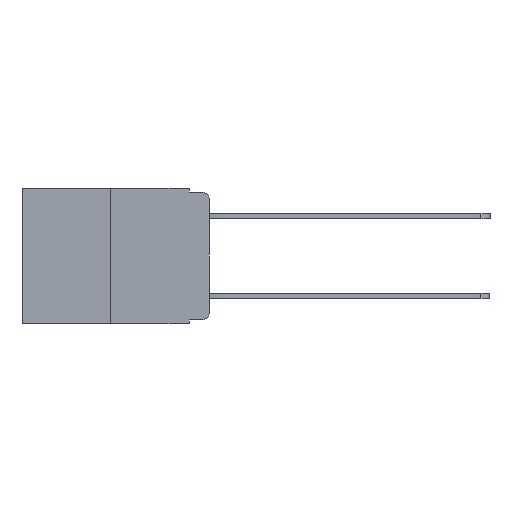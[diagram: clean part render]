
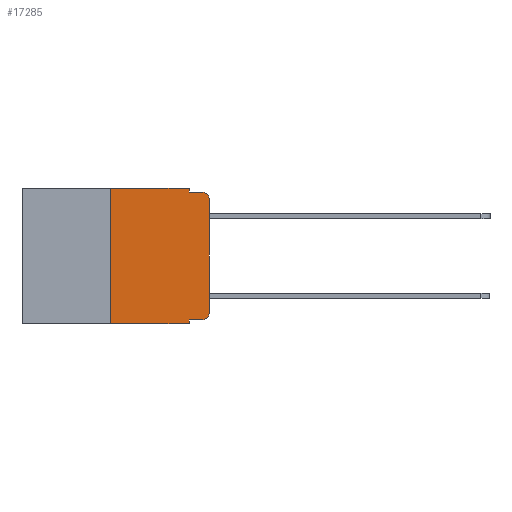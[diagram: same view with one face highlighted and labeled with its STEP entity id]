
A CAD part, left-side view. The second image highlights one B-rep face of the part: STEP entity #17285.
In plain terms, the highlighted planar face has unit normal (-1, 0, 0).
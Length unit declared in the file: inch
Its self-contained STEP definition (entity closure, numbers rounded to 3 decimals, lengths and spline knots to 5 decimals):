
#132 = DIRECTION ( 'NONE',  ( 0., -1., 0. ) ) ;
#447 = ORIENTED_EDGE ( 'NONE', *, *, #4931, .T. ) ;
#500 = VECTOR ( 'NONE', #19160, 39.37008 ) ;
#518 = CARTESIAN_POINT ( 'NONE',  ( 0., 0.02, -0.03 ) ) ;
#714 = ORIENTED_EDGE ( 'NONE', *, *, #6382, .F. ) ;
#965 = VERTEX_POINT ( 'NONE', #17814 ) ;
#993 = CARTESIAN_POINT ( 'NONE',  ( 0., 0.051, 0. ) ) ;
#1452 = VERTEX_POINT ( 'NONE', #8484 ) ;
#1464 = VECTOR ( 'NONE', #8050, 39.37008 ) ;
#2124 = ORIENTED_EDGE ( 'NONE', *, *, #16101, .T. ) ;
#2164 = DIRECTION ( 'NONE',  ( -1., 0., 0. ) ) ;
#2331 = DIRECTION ( 'NONE',  ( 0., 0., -1. ) ) ;
#3204 = EDGE_CURVE ( 'NONE', #4853, #1452, #14999, .T. ) ;
#3598 = LINE ( 'NONE', #10023, #22361 ) ;
#3828 = VERTEX_POINT ( 'NONE', #17256 ) ;
#4351 = ORIENTED_EDGE ( 'NONE', *, *, #3204, .F. ) ;
#4436 = CARTESIAN_POINT ( 'NONE',  ( 0., 0.051, 0. ) ) ;
#4838 = DIRECTION ( 'NONE',  ( 0., -1., 0. ) ) ;
#4853 = VERTEX_POINT ( 'NONE', #17505 ) ;
#4931 = EDGE_CURVE ( 'NONE', #15248, #3828, #8973, .T. ) ;
#4981 = CARTESIAN_POINT ( 'NONE',  ( 0., 0.473, 0. ) ) ;
#5122 = FACE_OUTER_BOUND ( 'NONE', #17758, .T. ) ;
#5472 = ORIENTED_EDGE ( 'NONE', *, *, #22164, .F. ) ;
#6382 = EDGE_CURVE ( 'NONE', #18717, #965, #17280, .T. ) ;
#7328 = CARTESIAN_POINT ( 'NONE',  ( 0., 0., 0. ) ) ;
#8050 = DIRECTION ( 'NONE',  ( 0., 0., -1. ) ) ;
#8475 = LINE ( 'NONE', #18452, #17084 ) ;
#8484 = CARTESIAN_POINT ( 'NONE',  ( 0., 0.02, -0.01 ) ) ;
#8698 = CARTESIAN_POINT ( 'NONE',  ( 0., 0.051, -0.333 ) ) ;
#8872 = DIRECTION ( 'NONE',  ( 1., 0., 0. ) ) ;
#8973 = CIRCLE ( 'NONE', #15539, 0.02 ) ;
#9043 = LINE ( 'NONE', #9268, #17649 ) ;
#9068 = DIRECTION ( 'NONE',  ( 0., 0., 1. ) ) ;
#9083 = EDGE_CURVE ( 'NONE', #17899, #19215, #9043, .T. ) ;
#9268 = CARTESIAN_POINT ( 'NONE',  ( 0., 0.473, -0.343 ) ) ;
#9529 = EDGE_CURVE ( 'NONE', #965, #4853, #22024, .T. ) ;
#10002 = EDGE_CURVE ( 'NONE', #10346, #1452, #13018, .T. ) ;
#10023 = CARTESIAN_POINT ( 'NONE',  ( 0., 0.051, -0.333 ) ) ;
#10346 = VERTEX_POINT ( 'NONE', #11925 ) ;
#10394 = VERTEX_POINT ( 'NONE', #8698 ) ;
#11460 = EDGE_CURVE ( 'NONE', #10394, #19215, #14855, .T. ) ;
#11925 = CARTESIAN_POINT ( 'NONE',  ( 0., 0., -0.03 ) ) ;
#12237 = ORIENTED_EDGE ( 'NONE', *, *, #9083, .T. ) ;
#12245 = PLANE ( 'NONE',  #21178 ) ;
#12425 = CARTESIAN_POINT ( 'NONE',  ( 0., 0.051, -0.01 ) ) ;
#12602 = CARTESIAN_POINT ( 'NONE',  ( 0., 0.02, -0.313 ) ) ;
#12766 = DIRECTION ( 'NONE',  ( -1., 0., 0. ) ) ;
#13018 = CIRCLE ( 'NONE', #15478, 0.02 ) ;
#13032 = ORIENTED_EDGE ( 'NONE', *, *, #10002, .T. ) ;
#13043 = VECTOR ( 'NONE', #18246, 39.37008 ) ;
#13574 = ORIENTED_EDGE ( 'NONE', *, *, #9529, .F. ) ;
#14342 = DIRECTION ( 'NONE',  ( 0., 0., -1. ) ) ;
#14855 = LINE ( 'NONE', #993, #1464 ) ;
#14999 = LINE ( 'NONE', #12425, #500 ) ;
#15248 = VERTEX_POINT ( 'NONE', #18218 ) ;
#15478 = AXIS2_PLACEMENT_3D ( 'NONE', #518, #12766, #2331 ) ;
#15539 = AXIS2_PLACEMENT_3D ( 'NONE', #12602, #2164, #14342 ) ;
#16101 = EDGE_CURVE ( 'NONE', #3828, #10346, #18107, .T. ) ;
#16918 = DIRECTION ( 'NONE',  ( 0., 0., 1. ) ) ;
#17084 = VECTOR ( 'NONE', #16918, 39.37008 ) ;
#17256 = CARTESIAN_POINT ( 'NONE',  ( 0., 0., -0.313 ) ) ;
#17280 = LINE ( 'NONE', #4981, #21190 ) ;
#17285 = ADVANCED_FACE ( 'NONE', ( #5122 ), #12245, .F. ) ;
#17447 = CARTESIAN_POINT ( 'NONE',  ( 0., 0.473, 0. ) ) ;
#17505 = CARTESIAN_POINT ( 'NONE',  ( 0., 0.051, -0.01 ) ) ;
#17649 = VECTOR ( 'NONE', #19562, 39.37008 ) ;
#17758 = EDGE_LOOP ( 'NONE', ( #2124, #13032, #4351, #13574, #714, #5472, #12237, #21758, #17887, #447 ) ) ;
#17814 = CARTESIAN_POINT ( 'NONE',  ( 0., 0.051, 0. ) ) ;
#17887 = ORIENTED_EDGE ( 'NONE', *, *, #20700, .T. ) ;
#17899 = VERTEX_POINT ( 'NONE', #22270 ) ;
#18107 = LINE ( 'NONE', #7328, #20437 ) ;
#18218 = CARTESIAN_POINT ( 'NONE',  ( 0., 0.02, -0.333 ) ) ;
#18246 = DIRECTION ( 'NONE',  ( 0., 0., -1. ) ) ;
#18452 = CARTESIAN_POINT ( 'NONE',  ( 0., 0.25, 0. ) ) ;
#18717 = VERTEX_POINT ( 'NONE', #19737 ) ;
#19160 = DIRECTION ( 'NONE',  ( 0., -1., 0. ) ) ;
#19215 = VERTEX_POINT ( 'NONE', #19354 ) ;
#19354 = CARTESIAN_POINT ( 'NONE',  ( 0., 0.051, -0.343 ) ) ;
#19562 = DIRECTION ( 'NONE',  ( 0., -1., 0. ) ) ;
#19737 = CARTESIAN_POINT ( 'NONE',  ( 0., 0.25, 0. ) ) ;
#20437 = VECTOR ( 'NONE', #9068, 39.37008 ) ;
#20700 = EDGE_CURVE ( 'NONE', #10394, #15248, #3598, .T. ) ;
#20768 = DIRECTION ( 'NONE',  ( 0., 0., -1. ) ) ;
#21178 = AXIS2_PLACEMENT_3D ( 'NONE', #17447, #8872, #20768 ) ;
#21190 = VECTOR ( 'NONE', #132, 39.37008 ) ;
#21758 = ORIENTED_EDGE ( 'NONE', *, *, #11460, .F. ) ;
#22024 = LINE ( 'NONE', #4436, #13043 ) ;
#22164 = EDGE_CURVE ( 'NONE', #17899, #18717, #8475, .T. ) ;
#22270 = CARTESIAN_POINT ( 'NONE',  ( 0., 0.25, -0.343 ) ) ;
#22361 = VECTOR ( 'NONE', #4838, 39.37008 ) ;
